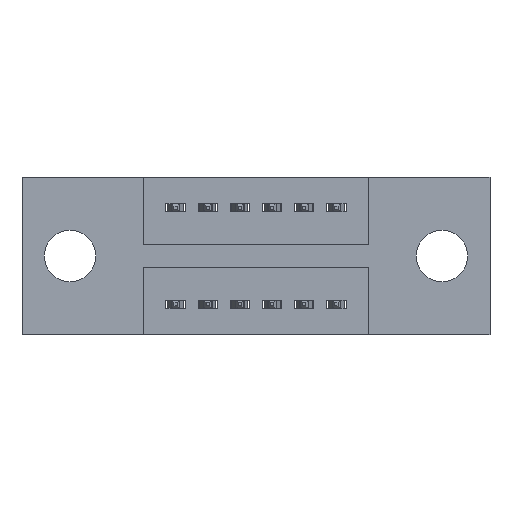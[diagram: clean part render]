
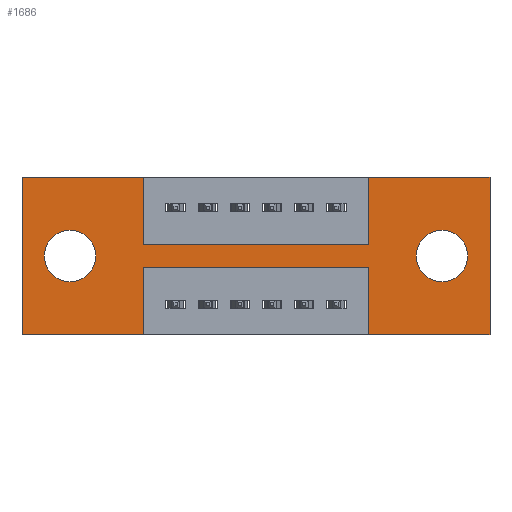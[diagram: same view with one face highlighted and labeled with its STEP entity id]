
A CAD part, front view. The second image highlights one B-rep face of the part: STEP entity #1686.
In plain terms, the highlighted planar face has unit normal (0, -1, 0).
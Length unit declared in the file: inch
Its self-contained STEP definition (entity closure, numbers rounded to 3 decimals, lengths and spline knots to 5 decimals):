
#13 = VERTEX_POINT ( 'NONE', #2819 ) ;
#32 = CARTESIAN_POINT ( 'NONE',  ( 1.455, 0., 0. ) ) ;
#134 = FACE_OUTER_BOUND ( 'NONE', #7716, .T. ) ;
#220 = DIRECTION ( 'NONE',  ( 1., 0., 0. ) ) ;
#299 = VECTOR ( 'NONE', #8298, 39.37008 ) ;
#348 = LINE ( 'NONE', #3653, #5929 ) ;
#354 = DIRECTION ( 'NONE',  ( 0., 0., 1. ) ) ;
#387 = CARTESIAN_POINT ( 'NONE',  ( 1.0775, 0., -0.21 ) ) ;
#641 = DIRECTION ( 'NONE',  ( 0., 1., 0. ) ) ;
#657 = VECTOR ( 'NONE', #2444, 39.37008 ) ;
#767 = LINE ( 'NONE', #5761, #657 ) ;
#961 = CARTESIAN_POINT ( 'NONE',  ( 0.3775, 0., -0.21 ) ) ;
#1003 = DIRECTION ( 'NONE',  ( 0., 0., -1. ) ) ;
#1037 = CARTESIAN_POINT ( 'NONE',  ( 0.3775, 0., -0.21 ) ) ;
#1070 = CARTESIAN_POINT ( 'NONE',  ( 0.3775, 0., -0.28 ) ) ;
#1175 = DIRECTION ( 'NONE',  ( 0., 1., 0. ) ) ;
#1209 = EDGE_CURVE ( 'NONE', #1275, #6583, #4161, .T. ) ;
#1275 = VERTEX_POINT ( 'NONE', #1762 ) ;
#1441 = LINE ( 'NONE', #961, #8076 ) ;
#1448 = CARTESIAN_POINT ( 'NONE',  ( 0., 0., 0. ) ) ;
#1449 = CARTESIAN_POINT ( 'NONE',  ( 0.1495, 0., -0.245 ) ) ;
#1496 = EDGE_CURVE ( 'NONE', #5255, #4656, #2378, .T. ) ;
#1571 = VERTEX_POINT ( 'NONE', #2247 ) ;
#1591 = EDGE_CURVE ( 'NONE', #6583, #5404, #348, .T. ) ;
#1620 = AXIS2_PLACEMENT_3D ( 'NONE', #1449, #4791, #2138 ) ;
#1644 = CARTESIAN_POINT ( 'NONE',  ( 0.3775, 0., -0.28 ) ) ;
#1673 = CARTESIAN_POINT ( 'NONE',  ( 1.455, 0., -0.49 ) ) ;
#1686 = ADVANCED_FACE ( 'NONE', ( #7786, #4575, #134 ), #3294, .T. ) ;
#1739 = VERTEX_POINT ( 'NONE', #5300 ) ;
#1762 = CARTESIAN_POINT ( 'NONE',  ( 1.0775, 0., 0. ) ) ;
#1966 = ORIENTED_EDGE ( 'NONE', *, *, #7548, .F. ) ;
#1968 = EDGE_CURVE ( 'NONE', #6678, #1739, #767, .T. ) ;
#2010 = ORIENTED_EDGE ( 'NONE', *, *, #3533, .F. ) ;
#2134 = LINE ( 'NONE', #2314, #299 ) ;
#2138 = DIRECTION ( 'NONE',  ( 0., 0., 1. ) ) ;
#2184 = CARTESIAN_POINT ( 'NONE',  ( 0., 0., -0.49 ) ) ;
#2195 = DIRECTION ( 'NONE',  ( 0., 0., 1. ) ) ;
#2247 = CARTESIAN_POINT ( 'NONE',  ( 0.3775, 0., -0.49 ) ) ;
#2255 = LINE ( 'NONE', #2184, #8291 ) ;
#2281 = ORIENTED_EDGE ( 'NONE', *, *, #6426, .T. ) ;
#2314 = CARTESIAN_POINT ( 'NONE',  ( 0., 0., 0. ) ) ;
#2366 = EDGE_CURVE ( 'NONE', #1571, #13, #2255, .T. ) ;
#2378 = CIRCLE ( 'NONE', #1620, 0.08 ) ;
#2406 = EDGE_CURVE ( 'NONE', #7461, #2491, #1441, .T. ) ;
#2444 = DIRECTION ( 'NONE',  ( 1., 0., 0. ) ) ;
#2491 = VERTEX_POINT ( 'NONE', #8395 ) ;
#2563 = DIRECTION ( 'NONE',  ( 0., 0., -1. ) ) ;
#2739 = DIRECTION ( 'NONE',  ( 0., -1., 0. ) ) ;
#2786 = VECTOR ( 'NONE', #5464, 39.37008 ) ;
#2798 = EDGE_CURVE ( 'NONE', #7383, #1571, #7853, .T. ) ;
#2814 = CIRCLE ( 'NONE', #5465, 0.08 ) ;
#2818 = ORIENTED_EDGE ( 'NONE', *, *, #7638, .T. ) ;
#2819 = CARTESIAN_POINT ( 'NONE',  ( 0., 0., -0.49 ) ) ;
#2993 = CARTESIAN_POINT ( 'NONE',  ( 0., 0., -0.49 ) ) ;
#3039 = LINE ( 'NONE', #2993, #7324 ) ;
#3152 = CARTESIAN_POINT ( 'NONE',  ( 0.3775, 0., -0.21 ) ) ;
#3168 = CARTESIAN_POINT ( 'NONE',  ( 1.3055, 0., -0.245 ) ) ;
#3187 = EDGE_CURVE ( 'NONE', #2491, #1275, #4331, .T. ) ;
#3275 = EDGE_LOOP ( 'NONE', ( #2281, #6875 ) ) ;
#3294 = PLANE ( 'NONE',  #4108 ) ;
#3326 = DIRECTION ( 'NONE',  ( 0., 0., -1. ) ) ;
#3533 = EDGE_CURVE ( 'NONE', #1739, #7461, #7139, .T. ) ;
#3653 = CARTESIAN_POINT ( 'NONE',  ( 1.455, 0., 0. ) ) ;
#3725 = CARTESIAN_POINT ( 'NONE',  ( 1.0775, 0., -0.28 ) ) ;
#4108 = AXIS2_PLACEMENT_3D ( 'NONE', #6013, #2739, #3326 ) ;
#4133 = EDGE_CURVE ( 'NONE', #13, #6678, #2134, .T. ) ;
#4151 = DIRECTION ( 'NONE',  ( 1., 0., 0. ) ) ;
#4161 = LINE ( 'NONE', #7471, #7784 ) ;
#4166 = CARTESIAN_POINT ( 'NONE',  ( 1.0775, 0., -0.28 ) ) ;
#4209 = CARTESIAN_POINT ( 'NONE',  ( 0.1495, 0., -0.245 ) ) ;
#4261 = ORIENTED_EDGE ( 'NONE', *, *, #6660, .F. ) ;
#4331 = LINE ( 'NONE', #387, #6406 ) ;
#4575 = FACE_BOUND ( 'NONE', #8360, .T. ) ;
#4656 = VERTEX_POINT ( 'NONE', #8411 ) ;
#4700 = VERTEX_POINT ( 'NONE', #3725 ) ;
#4708 = CARTESIAN_POINT ( 'NONE',  ( 1.0775, 0., -0.49 ) ) ;
#4788 = CARTESIAN_POINT ( 'NONE',  ( 0.1495, 0., -0.165 ) ) ;
#4791 = DIRECTION ( 'NONE',  ( 0., 1., 0. ) ) ;
#4827 = CARTESIAN_POINT ( 'NONE',  ( 0.3775, 0., -0.28 ) ) ;
#4863 = ORIENTED_EDGE ( 'NONE', *, *, #1209, .F. ) ;
#4934 = DIRECTION ( 'NONE',  ( 0., 1., 0. ) ) ;
#4950 = ORIENTED_EDGE ( 'NONE', *, *, #4133, .F. ) ;
#5009 = VERTEX_POINT ( 'NONE', #6820 ) ;
#5057 = EDGE_CURVE ( 'NONE', #5404, #6496, #3039, .T. ) ;
#5203 = LINE ( 'NONE', #4166, #5726 ) ;
#5255 = VERTEX_POINT ( 'NONE', #4788 ) ;
#5265 = ORIENTED_EDGE ( 'NONE', *, *, #1591, .F. ) ;
#5285 = CIRCLE ( 'NONE', #6172, 0.08 ) ;
#5300 = CARTESIAN_POINT ( 'NONE',  ( 0.3775, 0., 0. ) ) ;
#5404 = VERTEX_POINT ( 'NONE', #1673 ) ;
#5407 = ORIENTED_EDGE ( 'NONE', *, *, #1496, .T. ) ;
#5421 = ORIENTED_EDGE ( 'NONE', *, *, #1968, .F. ) ;
#5464 = DIRECTION ( 'NONE',  ( -1., 0., 0. ) ) ;
#5465 = AXIS2_PLACEMENT_3D ( 'NONE', #3168, #1175, #7823 ) ;
#5616 = DIRECTION ( 'NONE',  ( -1., 0., 0. ) ) ;
#5726 = VECTOR ( 'NONE', #2195, 39.37008 ) ;
#5738 = CARTESIAN_POINT ( 'NONE',  ( 1.3055, 0., -0.165 ) ) ;
#5761 = CARTESIAN_POINT ( 'NONE',  ( 0., 0., 0. ) ) ;
#5886 = DIRECTION ( 'NONE',  ( 0., 0., -1. ) ) ;
#5907 = ORIENTED_EDGE ( 'NONE', *, *, #2406, .F. ) ;
#5929 = VECTOR ( 'NONE', #2563, 39.37008 ) ;
#5946 = CARTESIAN_POINT ( 'NONE',  ( 1.3055, 0., -0.245 ) ) ;
#6013 = CARTESIAN_POINT ( 'NONE',  ( 0., 0., -0.49 ) ) ;
#6019 = VERTEX_POINT ( 'NONE', #5738 ) ;
#6172 = AXIS2_PLACEMENT_3D ( 'NONE', #4209, #4934, #354 ) ;
#6236 = ORIENTED_EDGE ( 'NONE', *, *, #2366, .F. ) ;
#6260 = DIRECTION ( 'NONE',  ( -1., 0., 0. ) ) ;
#6406 = VECTOR ( 'NONE', #8250, 39.37008 ) ;
#6413 = ORIENTED_EDGE ( 'NONE', *, *, #5057, .F. ) ;
#6426 = EDGE_CURVE ( 'NONE', #6019, #5009, #2814, .T. ) ;
#6496 = VERTEX_POINT ( 'NONE', #4708 ) ;
#6513 = VECTOR ( 'NONE', #1003, 39.37008 ) ;
#6583 = VERTEX_POINT ( 'NONE', #32 ) ;
#6660 = EDGE_CURVE ( 'NONE', #6496, #4700, #5203, .T. ) ;
#6678 = VERTEX_POINT ( 'NONE', #1448 ) ;
#6764 = ORIENTED_EDGE ( 'NONE', *, *, #2798, .F. ) ;
#6820 = CARTESIAN_POINT ( 'NONE',  ( 1.3055, 0., -0.325 ) ) ;
#6875 = ORIENTED_EDGE ( 'NONE', *, *, #8314, .T. ) ;
#7139 = LINE ( 'NONE', #1037, #6513 ) ;
#7324 = VECTOR ( 'NONE', #5616, 39.37008 ) ;
#7383 = VERTEX_POINT ( 'NONE', #1644 ) ;
#7415 = ORIENTED_EDGE ( 'NONE', *, *, #3187, .F. ) ;
#7461 = VERTEX_POINT ( 'NONE', #3152 ) ;
#7471 = CARTESIAN_POINT ( 'NONE',  ( 0., 0., 0. ) ) ;
#7479 = LINE ( 'NONE', #4827, #2786 ) ;
#7548 = EDGE_CURVE ( 'NONE', #4700, #7383, #7479, .T. ) ;
#7575 = CIRCLE ( 'NONE', #8059, 0.08 ) ;
#7638 = EDGE_CURVE ( 'NONE', #4656, #5255, #5285, .T. ) ;
#7651 = VECTOR ( 'NONE', #7746, 39.37008 ) ;
#7716 = EDGE_LOOP ( 'NONE', ( #7415, #5907, #2010, #5421, #4950, #6236, #6764, #1966, #4261, #6413, #5265, #4863 ) ) ;
#7746 = DIRECTION ( 'NONE',  ( 0., 0., -1. ) ) ;
#7784 = VECTOR ( 'NONE', #4151, 39.37008 ) ;
#7786 = FACE_BOUND ( 'NONE', #3275, .T. ) ;
#7823 = DIRECTION ( 'NONE',  ( 0., 0., -1. ) ) ;
#7853 = LINE ( 'NONE', #1070, #7651 ) ;
#8059 = AXIS2_PLACEMENT_3D ( 'NONE', #5946, #641, #5886 ) ;
#8076 = VECTOR ( 'NONE', #220, 39.37008 ) ;
#8250 = DIRECTION ( 'NONE',  ( 0., 0., 1. ) ) ;
#8291 = VECTOR ( 'NONE', #6260, 39.37008 ) ;
#8298 = DIRECTION ( 'NONE',  ( 0., 0., 1. ) ) ;
#8314 = EDGE_CURVE ( 'NONE', #5009, #6019, #7575, .T. ) ;
#8360 = EDGE_LOOP ( 'NONE', ( #5407, #2818 ) ) ;
#8395 = CARTESIAN_POINT ( 'NONE',  ( 1.0775, 0., -0.21 ) ) ;
#8411 = CARTESIAN_POINT ( 'NONE',  ( 0.1495, 0., -0.325 ) ) ;
